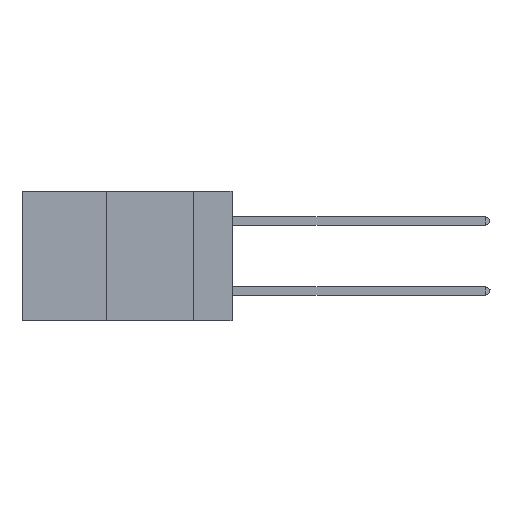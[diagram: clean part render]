
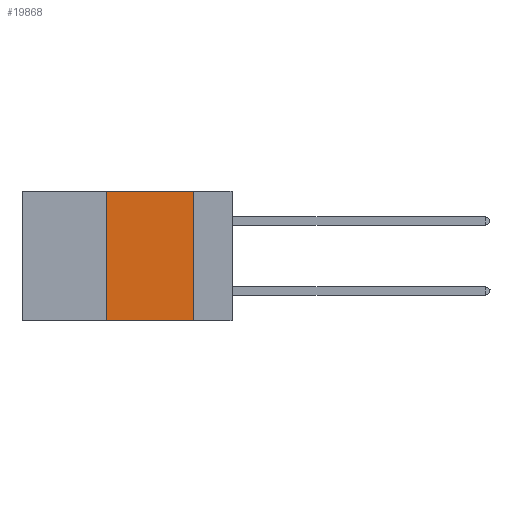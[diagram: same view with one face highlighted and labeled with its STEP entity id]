
A CAD part, left-side view. The second image highlights one B-rep face of the part: STEP entity #19868.
In plain terms, the highlighted planar face has unit normal (-1, 0, 0).
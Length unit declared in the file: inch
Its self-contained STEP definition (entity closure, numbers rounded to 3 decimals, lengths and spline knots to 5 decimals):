
#102 = DIRECTION ( 'NONE',  ( 0., 0., -1. ) ) ;
#339 = PLANE ( 'NONE',  #10275 ) ;
#408 = VERTEX_POINT ( 'NONE', #17294 ) ;
#1625 = VECTOR ( 'NONE', #16563, 39.37008 ) ;
#2909 = EDGE_CURVE ( 'NONE', #10807, #408, #16668, .T. ) ;
#3790 = ORIENTED_EDGE ( 'NONE', *, *, #20935, .F. ) ;
#6234 = CARTESIAN_POINT ( 'NONE',  ( 0., 0.11, 0. ) ) ;
#7980 = DIRECTION ( 'NONE',  ( 0., 0., -1. ) ) ;
#8276 = VECTOR ( 'NONE', #14384, 39.37008 ) ;
#9339 = CARTESIAN_POINT ( 'NONE',  ( 0., 0.6, -0.37 ) ) ;
#9476 = VECTOR ( 'NONE', #22021, 39.37008 ) ;
#9501 = CARTESIAN_POINT ( 'NONE',  ( 0., 0.36, 0. ) ) ;
#9522 = DIRECTION ( 'NONE',  ( 1., 0., 0. ) ) ;
#10035 = ORIENTED_EDGE ( 'NONE', *, *, #14062, .T. ) ;
#10275 = AXIS2_PLACEMENT_3D ( 'NONE', #16742, #9522, #102 ) ;
#10807 = VERTEX_POINT ( 'NONE', #14144 ) ;
#11897 = VERTEX_POINT ( 'NONE', #22994 ) ;
#12462 = CARTESIAN_POINT ( 'NONE',  ( 0., 0.6, 0. ) ) ;
#14062 = EDGE_CURVE ( 'NONE', #10807, #19109, #22150, .T. ) ;
#14144 = CARTESIAN_POINT ( 'NONE',  ( 0., 0.36, -0.37 ) ) ;
#14157 = LINE ( 'NONE', #6234, #14436 ) ;
#14384 = DIRECTION ( 'NONE',  ( 0., -1., 0. ) ) ;
#14436 = VECTOR ( 'NONE', #7980, 39.37008 ) ;
#14473 = CARTESIAN_POINT ( 'NONE',  ( 0., 0.11, -0.37 ) ) ;
#14688 = ORIENTED_EDGE ( 'NONE', *, *, #2909, .F. ) ;
#16563 = DIRECTION ( 'NONE',  ( 0., 0., 1. ) ) ;
#16668 = LINE ( 'NONE', #9501, #1625 ) ;
#16742 = CARTESIAN_POINT ( 'NONE',  ( 0., 0.6, 0. ) ) ;
#17093 = ORIENTED_EDGE ( 'NONE', *, *, #17184, .F. ) ;
#17103 = FACE_OUTER_BOUND ( 'NONE', #19081, .T. ) ;
#17184 = EDGE_CURVE ( 'NONE', #11897, #19109, #14157, .T. ) ;
#17294 = CARTESIAN_POINT ( 'NONE',  ( 0., 0.36, 0. ) ) ;
#19081 = EDGE_LOOP ( 'NONE', ( #17093, #3790, #14688, #10035 ) ) ;
#19109 = VERTEX_POINT ( 'NONE', #14473 ) ;
#19868 = ADVANCED_FACE ( 'NONE', ( #17103 ), #339, .F. ) ;
#20437 = LINE ( 'NONE', #12462, #8276 ) ;
#20935 = EDGE_CURVE ( 'NONE', #408, #11897, #20437, .T. ) ;
#22021 = DIRECTION ( 'NONE',  ( 0., -1., 0. ) ) ;
#22150 = LINE ( 'NONE', #9339, #9476 ) ;
#22994 = CARTESIAN_POINT ( 'NONE',  ( 0., 0.11, 0. ) ) ;
